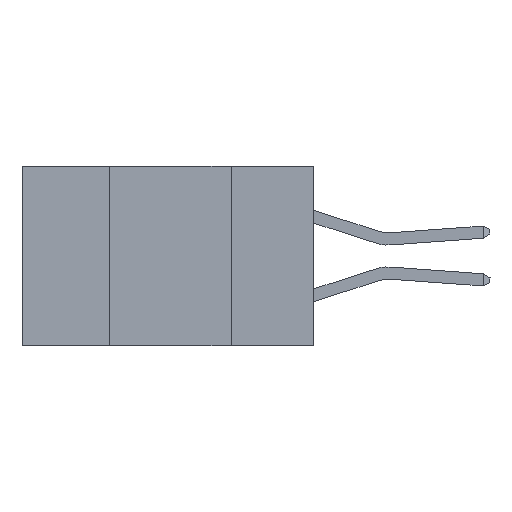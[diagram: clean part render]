
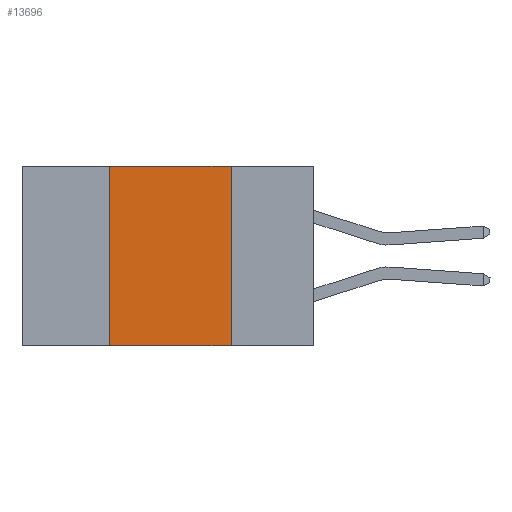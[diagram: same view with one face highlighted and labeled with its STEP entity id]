
A CAD part, left-side view. The second image highlights one B-rep face of the part: STEP entity #13696.
In plain terms, the highlighted planar face has unit normal (-1, 0, 0).
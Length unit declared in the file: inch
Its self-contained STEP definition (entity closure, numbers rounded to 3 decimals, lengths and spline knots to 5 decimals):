
#369 = EDGE_CURVE ( 'NONE', #20638, #20958, #12768, .T. ) ;
#1669 = FACE_OUTER_BOUND ( 'NONE', #11465, .T. ) ;
#3706 = CARTESIAN_POINT ( 'NONE',  ( 0., 0.17, 0. ) ) ;
#4829 = VERTEX_POINT ( 'NONE', #14498 ) ;
#4963 = LINE ( 'NONE', #6824, #14438 ) ;
#4990 = CARTESIAN_POINT ( 'NONE',  ( 0., 0.17, -0.37 ) ) ;
#5967 = DIRECTION ( 'NONE',  ( 0., 0., 1. ) ) ;
#6824 = CARTESIAN_POINT ( 'NONE',  ( 0., 0.6, 0. ) ) ;
#6941 = DIRECTION ( 'NONE',  ( 0., -1., 0. ) ) ;
#7141 = ORIENTED_EDGE ( 'NONE', *, *, #22619, .F. ) ;
#7663 = DIRECTION ( 'NONE',  ( 1., 0., 0. ) ) ;
#9080 = ORIENTED_EDGE ( 'NONE', *, *, #369, .F. ) ;
#9287 = PLANE ( 'NONE',  #21842 ) ;
#9748 = CARTESIAN_POINT ( 'NONE',  ( 0., 0.17, 0. ) ) ;
#9845 = VECTOR ( 'NONE', #11288, 39.37008 ) ;
#10882 = CARTESIAN_POINT ( 'NONE',  ( 0., 0.42, -0.37 ) ) ;
#11288 = DIRECTION ( 'NONE',  ( 0., 0., -1. ) ) ;
#11300 = LINE ( 'NONE', #18960, #17493 ) ;
#11465 = EDGE_LOOP ( 'NONE', ( #9080, #7141, #20398, #23820 ) ) ;
#12768 = LINE ( 'NONE', #3706, #9845 ) ;
#13696 = ADVANCED_FACE ( 'NONE', ( #1669 ), #9287, .F. ) ;
#13967 = VECTOR ( 'NONE', #24507, 39.37008 ) ;
#14438 = VECTOR ( 'NONE', #6941, 39.37008 ) ;
#14498 = CARTESIAN_POINT ( 'NONE',  ( 0., 0.42, 0. ) ) ;
#15242 = DIRECTION ( 'NONE',  ( 0., 0., -1. ) ) ;
#16394 = EDGE_CURVE ( 'NONE', #17696, #20958, #22529, .T. ) ;
#16939 = CARTESIAN_POINT ( 'NONE',  ( 0., 0.6, -0.37 ) ) ;
#17493 = VECTOR ( 'NONE', #5967, 39.37008 ) ;
#17696 = VERTEX_POINT ( 'NONE', #10882 ) ;
#18960 = CARTESIAN_POINT ( 'NONE',  ( 0., 0.42, 0. ) ) ;
#19147 = EDGE_CURVE ( 'NONE', #17696, #4829, #11300, .T. ) ;
#20398 = ORIENTED_EDGE ( 'NONE', *, *, #19147, .F. ) ;
#20638 = VERTEX_POINT ( 'NONE', #9748 ) ;
#20958 = VERTEX_POINT ( 'NONE', #4990 ) ;
#21842 = AXIS2_PLACEMENT_3D ( 'NONE', #22662, #7663, #15242 ) ;
#22529 = LINE ( 'NONE', #16939, #13967 ) ;
#22619 = EDGE_CURVE ( 'NONE', #4829, #20638, #4963, .T. ) ;
#22662 = CARTESIAN_POINT ( 'NONE',  ( 0., 0.6, 0. ) ) ;
#23820 = ORIENTED_EDGE ( 'NONE', *, *, #16394, .T. ) ;
#24507 = DIRECTION ( 'NONE',  ( 0., -1., 0. ) ) ;
